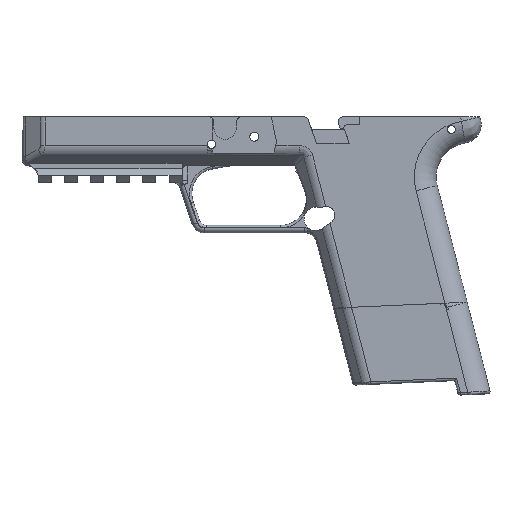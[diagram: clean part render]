
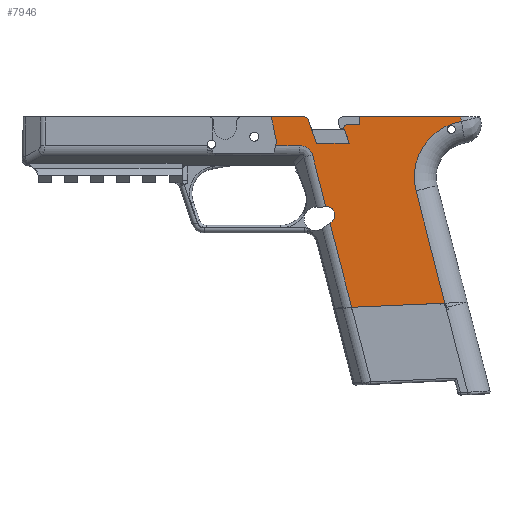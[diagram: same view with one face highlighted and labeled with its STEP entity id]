
A CAD part, left-side view. The second image highlights one B-rep face of the part: STEP entity #7946.
In plain terms, the highlighted face is planar.
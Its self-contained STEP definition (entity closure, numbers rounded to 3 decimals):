
#209=CIRCLE('',#8516,1.);
#210=CIRCLE('',#8518,2.);
#211=CIRCLE('',#8520,3.585);
#212=CIRCLE('',#8521,2.921);
#213=CIRCLE('',#8522,3.585);
#214=CIRCLE('',#8523,22.475);
#215=CIRCLE('',#8524,7.5);
#661=FACE_OUTER_BOUND('',#1109,.T.);
#1109=EDGE_LOOP('',(#5927,#5928,#5929,#5930,#5931,#5932,#5933,#5934,#5935,
#5936,#5937,#5938,#5939,#5940,#5941,#5942,#5943,#5944,#5945,#5946,#5947,
#5948,#5949));
#1682=LINE('',#13142,#2413);
#1683=LINE('',#13144,#2414);
#1684=LINE('',#13146,#2415);
#1685=LINE('',#13150,#2416);
#1686=LINE('',#13152,#2417);
#1687=LINE('',#13154,#2418);
#1688=LINE('',#13156,#2419);
#1689=LINE('',#13160,#2420);
#1690=LINE('',#13168,#2421);
#1691=LINE('',#13170,#2422);
#1692=LINE('',#13172,#2423);
#1693=LINE('',#13174,#2424);
#1694=LINE('',#13180,#2425);
#1695=LINE('',#13182,#2426);
#1696=LINE('',#13183,#2427);
#2413=VECTOR('',#9790,10.);
#2414=VECTOR('',#9791,10.);
#2415=VECTOR('',#9792,10.);
#2416=VECTOR('',#9795,10.);
#2417=VECTOR('',#9796,10.);
#2418=VECTOR('',#9797,10.);
#2419=VECTOR('',#9798,10.);
#2420=VECTOR('',#9801,10.);
#2421=VECTOR('',#9808,10.);
#2422=VECTOR('',#9809,10.);
#2423=VECTOR('',#9810,10.);
#2424=VECTOR('',#9811,10.);
#2425=VECTOR('',#9816,10.);
#2426=VECTOR('',#9817,10.);
#2427=VECTOR('',#9818,10.);
#2928=ELLIPSE('',#8519,10.693,7.);
#3441=VERTEX_POINT('',#13135);
#3442=VERTEX_POINT('',#13137);
#3443=VERTEX_POINT('',#13141);
#3444=VERTEX_POINT('',#13143);
#3445=VERTEX_POINT('',#13145);
#3446=VERTEX_POINT('',#13147);
#3447=VERTEX_POINT('',#13149);
#3448=VERTEX_POINT('',#13151);
#3449=VERTEX_POINT('',#13153);
#3450=VERTEX_POINT('',#13155);
#3451=VERTEX_POINT('',#13157);
#3452=VERTEX_POINT('',#13159);
#3453=VERTEX_POINT('',#13161);
#3454=VERTEX_POINT('',#13163);
#3455=VERTEX_POINT('',#13165);
#3456=VERTEX_POINT('',#13167);
#3457=VERTEX_POINT('',#13169);
#3458=VERTEX_POINT('',#13171);
#3459=VERTEX_POINT('',#13173);
#3460=VERTEX_POINT('',#13175);
#3461=VERTEX_POINT('',#13177);
#3462=VERTEX_POINT('',#13179);
#3463=VERTEX_POINT('',#13181);
#4356=EDGE_CURVE('',#3441,#3442,#209,.T.);
#4358=EDGE_CURVE('',#3441,#3443,#1682,.F.);
#4359=EDGE_CURVE('',#3443,#3444,#1683,.T.);
#4360=EDGE_CURVE('',#3444,#3445,#1684,.F.);
#4361=EDGE_CURVE('',#3446,#3445,#210,.T.);
#4362=EDGE_CURVE('',#3446,#3447,#1685,.T.);
#4363=EDGE_CURVE('',#3447,#3448,#1686,.T.);
#4364=EDGE_CURVE('',#3448,#3449,#1687,.T.);
#4365=EDGE_CURVE('',#3450,#3449,#1688,.T.);
#4366=EDGE_CURVE('',#3451,#3450,#2928,.T.);
#4367=EDGE_CURVE('',#3452,#3451,#1689,.T.);
#4368=EDGE_CURVE('',#3452,#3453,#211,.T.);
#4369=EDGE_CURVE('',#3453,#3454,#212,.T.);
#4370=EDGE_CURVE('',#3454,#3455,#213,.T.);
#4371=EDGE_CURVE('',#3455,#3456,#1690,.T.);
#4372=EDGE_CURVE('',#3457,#3456,#1691,.T.);
#4373=EDGE_CURVE('',#3458,#3457,#1692,.T.);
#4374=EDGE_CURVE('',#3459,#3458,#1693,.T.);
#4375=EDGE_CURVE('',#3460,#3459,#214,.T.);
#4376=EDGE_CURVE('',#3461,#3460,#215,.T.);
#4377=EDGE_CURVE('',#3461,#3462,#1694,.T.);
#4378=EDGE_CURVE('',#3462,#3463,#1695,.F.);
#4379=EDGE_CURVE('',#3463,#3442,#1696,.T.);
#5927=ORIENTED_EDGE('',*,*,#4356,.F.);
#5928=ORIENTED_EDGE('',*,*,#4358,.T.);
#5929=ORIENTED_EDGE('',*,*,#4359,.T.);
#5930=ORIENTED_EDGE('',*,*,#4360,.T.);
#5931=ORIENTED_EDGE('',*,*,#4361,.F.);
#5932=ORIENTED_EDGE('',*,*,#4362,.T.);
#5933=ORIENTED_EDGE('',*,*,#4363,.T.);
#5934=ORIENTED_EDGE('',*,*,#4364,.T.);
#5935=ORIENTED_EDGE('',*,*,#4365,.F.);
#5936=ORIENTED_EDGE('',*,*,#4366,.F.);
#5937=ORIENTED_EDGE('',*,*,#4367,.F.);
#5938=ORIENTED_EDGE('',*,*,#4368,.T.);
#5939=ORIENTED_EDGE('',*,*,#4369,.T.);
#5940=ORIENTED_EDGE('',*,*,#4370,.T.);
#5941=ORIENTED_EDGE('',*,*,#4371,.T.);
#5942=ORIENTED_EDGE('',*,*,#4372,.F.);
#5943=ORIENTED_EDGE('',*,*,#4373,.F.);
#5944=ORIENTED_EDGE('',*,*,#4374,.F.);
#5945=ORIENTED_EDGE('',*,*,#4375,.F.);
#5946=ORIENTED_EDGE('',*,*,#4376,.F.);
#5947=ORIENTED_EDGE('',*,*,#4377,.T.);
#5948=ORIENTED_EDGE('',*,*,#4378,.T.);
#5949=ORIENTED_EDGE('',*,*,#4379,.T.);
#7658=PLANE('',#8517);
#7946=ADVANCED_FACE('',(#661),#7658,.F.);
#8516=AXIS2_PLACEMENT_3D('',#13138,#9785,#9786);
#8517=AXIS2_PLACEMENT_3D('',#13140,#9788,#9789);
#8518=AXIS2_PLACEMENT_3D('',#13148,#9793,#9794);
#8519=AXIS2_PLACEMENT_3D('',#13158,#9799,#9800);
#8520=AXIS2_PLACEMENT_3D('',#13162,#9802,#9803);
#8521=AXIS2_PLACEMENT_3D('',#13164,#9804,#9805);
#8522=AXIS2_PLACEMENT_3D('',#13166,#9806,#9807);
#8523=AXIS2_PLACEMENT_3D('',#13176,#9812,#9813);
#8524=AXIS2_PLACEMENT_3D('',#13178,#9814,#9815);
#9785=DIRECTION('center_axis',(-1.,0.,0.));
#9786=DIRECTION('ref_axis',(0.,0.817,-0.576));
#9788=DIRECTION('center_axis',(-1.,0.,0.));
#9789=DIRECTION('ref_axis',(0.,1.,0.));
#9790=DIRECTION('',(0.,0.336,-0.942));
#9791=DIRECTION('',(0.,1.,0.));
#9792=DIRECTION('',(0.,-0.336,0.942));
#9793=DIRECTION('center_axis',(-1.,0.,0.));
#9794=DIRECTION('ref_axis',(0.,-0.576,-0.817));
#9795=DIRECTION('',(0.,1.,0.));
#9796=DIRECTION('',(0.,-0.21,0.978));
#9797=DIRECTION('',(0.,0.21,0.978));
#9798=DIRECTION('',(0.,1.,0.));
#9799=DIRECTION('center_axis',(1.,0.,0.));
#9800=DIRECTION('ref_axis',(0.,-0.714,-0.7));
#9801=DIRECTION('',(0.,0.249,-0.969));
#9802=DIRECTION('center_axis',(-1.,0.,0.));
#9803=DIRECTION('ref_axis',(0.,1.,0.));
#9804=DIRECTION('center_axis',(-1.,0.,0.));
#9805=DIRECTION('ref_axis',(0.,1.,0.));
#9806=DIRECTION('center_axis',(-1.,0.,0.));
#9807=DIRECTION('ref_axis',(0.,1.,0.));
#9808=DIRECTION('',(0.,0.828,0.56));
#9809=DIRECTION('',(0.,0.249,-0.969));
#9810=DIRECTION('',(0.,0.999,0.044));
#9811=DIRECTION('',(0.,-0.249,0.969));
#9812=DIRECTION('center_axis',(1.,0.,0.));
#9813=DIRECTION('ref_axis',(0.,0.,1.));
#9814=DIRECTION('center_axis',(1.,0.,0.));
#9815=DIRECTION('ref_axis',(0.,-0.97,-0.244));
#9816=DIRECTION('',(0.,1.,0.));
#9817=DIRECTION('',(0.,0.,-1.));
#9818=DIRECTION('',(0.,1.,0.));
#13135=CARTESIAN_POINT('',(22.175,-34.374,-2.995));
#13137=CARTESIAN_POINT('',(22.175,-35.316,-4.331));
#13138=CARTESIAN_POINT('Origin',(22.175,-35.316,-3.331));
#13140=CARTESIAN_POINT('Origin',(22.175,-7.921,2.186));
#13141=CARTESIAN_POINT('',(22.175,-36.514,3.));
#13142=CARTESIAN_POINT('',(22.175,-32.976,-6.913));
#13143=CARTESIAN_POINT('',(22.175,-23.407,3.));
#13144=CARTESIAN_POINT('',(22.175,-23.764,3.));
#13145=CARTESIAN_POINT('',(22.175,-20.114,-6.228));
#13146=CARTESIAN_POINT('',(22.175,-21.552,-2.199));
#13147=CARTESIAN_POINT('',(22.175,-18.23,-7.556));
#13148=CARTESIAN_POINT('Origin',(22.175,-18.23,-5.556));
#13149=CARTESIAN_POINT('',(22.175,-5.3,-7.556));
#13150=CARTESIAN_POINT('',(22.175,-86.951,-7.556));
#13151=CARTESIAN_POINT('',(22.175,-7.389,2.186));
#13152=CARTESIAN_POINT('',(22.175,-6.356,-2.63));
#13153=CARTESIAN_POINT('',(22.175,-7.025,3.884));
#13154=CARTESIAN_POINT('',(22.175,-7.4,2.132));
#13155=CARTESIAN_POINT('',(22.175,-16.536,3.884));
#13156=CARTESIAN_POINT('',(22.175,33.814,3.884));
#13157=CARTESIAN_POINT('',(22.175,-21.783,7.651));
#13158=CARTESIAN_POINT('Origin',(22.175,-12.907,12.884));
#13159=CARTESIAN_POINT('',(22.175,-27.074,28.233));
#13160=CARTESIAN_POINT('',(22.175,-26.659,26.619));
#13161=CARTESIAN_POINT('',(22.175,-30.502,30.561));
#13162=CARTESIAN_POINT('Origin',(22.175,-27.144,31.817));
#13163=CARTESIAN_POINT('',(22.175,-30.617,30.925));
#13164=CARTESIAN_POINT('Origin',(22.175,-27.779,31.618));
#13165=CARTESIAN_POINT('',(22.175,-29.153,34.787));
#13166=CARTESIAN_POINT('Origin',(22.175,-27.144,31.817));
#13167=CARTESIAN_POINT('',(22.175,-28.817,35.014));
#13168=CARTESIAN_POINT('',(22.175,-27.054,36.207));
#13169=CARTESIAN_POINT('',(22.175,-37.447,68.587));
#13170=CARTESIAN_POINT('',(22.175,-26.659,26.619));
#13171=CARTESIAN_POINT('',(22.175,-74.722,66.935));
#13172=CARTESIAN_POINT('',(22.175,-40.785,68.439));
#13173=CARTESIAN_POINT('',(22.175,-63.184,22.049));
#13174=CARTESIAN_POINT('',(22.175,-75.103,68.418));
#13175=CARTESIAN_POINT('',(22.175,-81.332,-5.728));
#13176=CARTESIAN_POINT('Origin',(22.175,-84.951,16.453));
#13177=CARTESIAN_POINT('',(22.175,-81.106,-7.556));
#13178=CARTESIAN_POINT('Origin',(22.175,-88.606,-7.556));
#13179=CARTESIAN_POINT('',(22.175,-40.774,-7.556));
#13180=CARTESIAN_POINT('',(22.175,-84.951,-7.556));
#13181=CARTESIAN_POINT('',(22.175,-40.774,-4.331));
#13182=CARTESIAN_POINT('',(22.175,-40.774,-2.685));
#13183=CARTESIAN_POINT('',(22.175,-20.598,-4.331));
